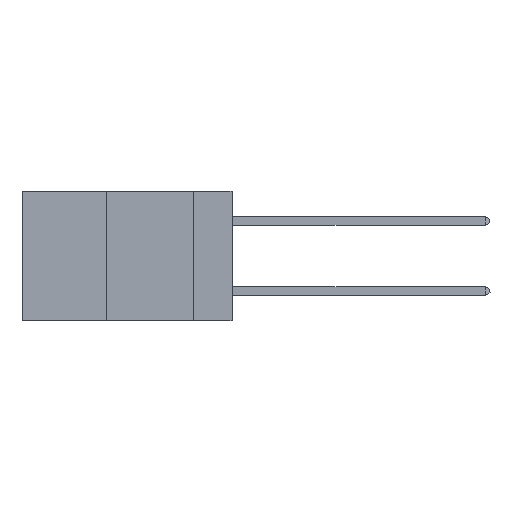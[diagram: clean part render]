
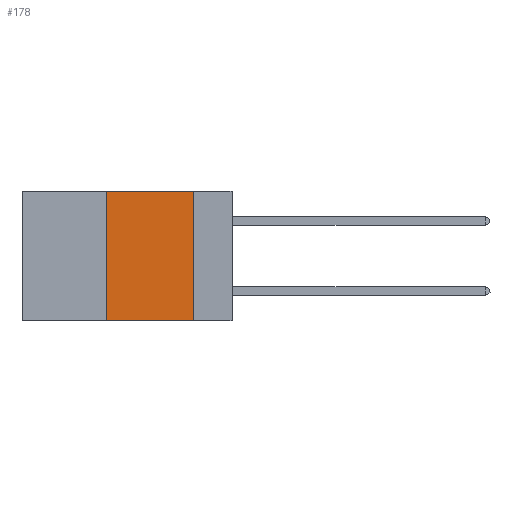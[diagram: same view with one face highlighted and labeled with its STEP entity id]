
A CAD part, left-side view. The second image highlights one B-rep face of the part: STEP entity #178.
In plain terms, the highlighted planar face has unit normal (-1, 0, 0).
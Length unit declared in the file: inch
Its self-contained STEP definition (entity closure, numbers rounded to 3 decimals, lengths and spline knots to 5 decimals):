
#20 = DIRECTION ( 'NONE',  ( 1., 0., 0. ) ) ;
#178 = ADVANCED_FACE ( 'NONE', ( #7378 ), #4047, .F. ) ;
#245 = CARTESIAN_POINT ( 'NONE',  ( 0., 0.6, -0.37 ) ) ;
#314 = AXIS2_PLACEMENT_3D ( 'NONE', #7325, #20, #3256 ) ;
#738 = VERTEX_POINT ( 'NONE', #10168 ) ;
#1674 = EDGE_CURVE ( 'NONE', #738, #8455, #2684, .T. ) ;
#1847 = CARTESIAN_POINT ( 'NONE',  ( 0., 0.11, 0. ) ) ;
#2082 = DIRECTION ( 'NONE',  ( 0., -1., 0. ) ) ;
#2684 = LINE ( 'NONE', #4376, #9818 ) ;
#3256 = DIRECTION ( 'NONE',  ( 0., 0., -1. ) ) ;
#3535 = ORIENTED_EDGE ( 'NONE', *, *, #7348, .F. ) ;
#3831 = VERTEX_POINT ( 'NONE', #8186 ) ;
#4047 = PLANE ( 'NONE',  #314 ) ;
#4102 = VECTOR ( 'NONE', #2082, 39.37008 ) ;
#4376 = CARTESIAN_POINT ( 'NONE',  ( 0., 0.36, 0. ) ) ;
#5005 = CARTESIAN_POINT ( 'NONE',  ( 0., 0.11, 0. ) ) ;
#5193 = EDGE_CURVE ( 'NONE', #8455, #9647, #7816, .T. ) ;
#5204 = LINE ( 'NONE', #5005, #8003 ) ;
#5952 = DIRECTION ( 'NONE',  ( 0., -1., 0. ) ) ;
#6006 = CARTESIAN_POINT ( 'NONE',  ( 0., 0.36, 0. ) ) ;
#6333 = EDGE_LOOP ( 'NONE', ( #3535, #6957, #7577, #7608 ) ) ;
#6392 = LINE ( 'NONE', #245, #8497 ) ;
#6957 = ORIENTED_EDGE ( 'NONE', *, *, #5193, .F. ) ;
#7325 = CARTESIAN_POINT ( 'NONE',  ( 0., 0.6, 0. ) ) ;
#7348 = EDGE_CURVE ( 'NONE', #9647, #3831, #5204, .T. ) ;
#7378 = FACE_OUTER_BOUND ( 'NONE', #6333, .T. ) ;
#7577 = ORIENTED_EDGE ( 'NONE', *, *, #1674, .F. ) ;
#7608 = ORIENTED_EDGE ( 'NONE', *, *, #7641, .T. ) ;
#7641 = EDGE_CURVE ( 'NONE', #738, #3831, #6392, .T. ) ;
#7690 = DIRECTION ( 'NONE',  ( 0., 0., -1. ) ) ;
#7816 = LINE ( 'NONE', #7988, #4102 ) ;
#7988 = CARTESIAN_POINT ( 'NONE',  ( 0., 0.6, 0. ) ) ;
#8003 = VECTOR ( 'NONE', #7690, 39.37008 ) ;
#8186 = CARTESIAN_POINT ( 'NONE',  ( 0., 0.11, -0.37 ) ) ;
#8455 = VERTEX_POINT ( 'NONE', #6006 ) ;
#8497 = VECTOR ( 'NONE', #5952, 39.37008 ) ;
#9280 = DIRECTION ( 'NONE',  ( 0., 0., 1. ) ) ;
#9647 = VERTEX_POINT ( 'NONE', #1847 ) ;
#9818 = VECTOR ( 'NONE', #9280, 39.37008 ) ;
#10168 = CARTESIAN_POINT ( 'NONE',  ( 0., 0.36, -0.37 ) ) ;
